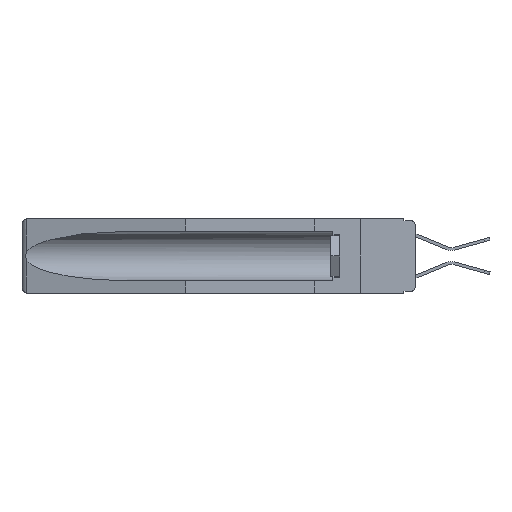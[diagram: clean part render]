
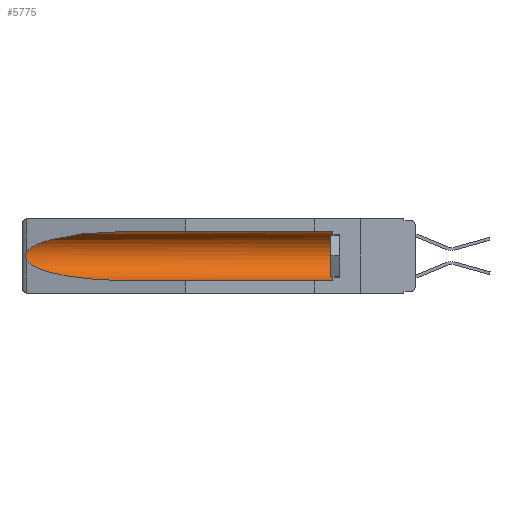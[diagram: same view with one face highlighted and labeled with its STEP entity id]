
A CAD part, left-side view. The second image highlights one B-rep face of the part: STEP entity #5775.
In plain terms, the highlighted cylindrical face has radius 2.857 mm (diameter 5.715 mm), a partial arc.
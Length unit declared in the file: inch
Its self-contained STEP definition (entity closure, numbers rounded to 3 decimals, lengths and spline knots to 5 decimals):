
#430 = VECTOR ( 'NONE', #15503, 39.37008 ) ;
#991 = DIRECTION ( 'NONE',  ( 0., 1., 0. ) ) ;
#1153 = CARTESIAN_POINT ( 'NONE',  ( 0.26537, 1.52718, -0.14972 ) ) ;
#1721 = CARTESIAN_POINT ( 'NONE',  ( 0.2675, 1.53308, -0.16763 ) ) ;
#1985 = DIRECTION ( 'NONE',  ( 0., 0., 1. ) ) ;
#2194 = ORIENTED_EDGE ( 'NONE', *, *, #4719, .T. ) ;
#2524 = VERTEX_POINT ( 'NONE', #5177 ) ;
#2529 = VERTEX_POINT ( 'NONE', #14973 ) ;
#2589 = VECTOR ( 'NONE', #991, 39.37008 ) ;
#3140 = CARTESIAN_POINT ( 'NONE',  ( 0.26597, 1.5296, -0.19026 ) ) ;
#3975 = FACE_OUTER_BOUND ( 'NONE', #15320, .T. ) ;
#4367 = CARTESIAN_POINT ( 'NONE',  ( 0.155, -0.30754, -0.284 ) ) ;
#4464 = CARTESIAN_POINT ( 'NONE',  ( 0.155, -0.30754, -0.059 ) ) ;
#4719 = EDGE_CURVE ( 'NONE', #2524, #11640, #8384, .T. ) ;
#4727 = LINE ( 'NONE', #4367, #430 ) ;
#5177 = CARTESIAN_POINT ( 'NONE',  ( 0.155, 1.07973, -0.059 ) ) ;
#5775 = ADVANCED_FACE ( 'NONE', ( #3975 ), #19039, .F. ) ;
#5971 = EDGE_CURVE ( 'NONE', #19521, #2529, #4727, .T. ) ;
#6117 = CARTESIAN_POINT ( 'NONE',  ( 0.155, -0.30754, -0.1715 ) ) ;
#6275 = CARTESIAN_POINT ( 'NONE',  ( 0.26655, 1.53094, -0.18657 ) ) ;
#6411 = CARTESIAN_POINT ( 'NONE',  ( 0.26597, 1.52961, -0.15275 ) ) ;
#6857 = CARTESIAN_POINT ( 'NONE',  ( 0.155, 0.126, -0.1715 ) ) ;
#6981 = EDGE_CURVE ( 'NONE', #19657, #2529, #10424, .T. ) ;
#8384 =( BOUNDED_CURVE ( )  B_SPLINE_CURVE ( 3, ( #14329, #19924, #10711, #1153 ),
 .UNSPECIFIED., .F., .F. ) 
 B_SPLINE_CURVE_WITH_KNOTS ( ( 4, 4 ),
 ( 4.71239, 6.08839 ),
 .UNSPECIFIED. ) 
 CURVE ( )  GEOMETRIC_REPRESENTATION_ITEM ( )  RATIONAL_B_SPLINE_CURVE ( ( 1., 0.848, 0.848, 1. ) ) 
 REPRESENTATION_ITEM ( '' )  );
#8856 = LINE ( 'NONE', #4464, #2589 ) ;
#9444 = CARTESIAN_POINT ( 'NONE',  ( 0.26537, 1.52718, -0.19328 ) ) ;
#9794 = B_SPLINE_CURVE_WITH_KNOTS ( 'NONE', 3,
 ( #15824, #6411, #12752, #19208, #1721, #19073, #12892, #6275, #3140, #9444 ),
 .UNSPECIFIED., .F., .F.,
 ( 4, 2, 2, 2, 4 ),
 ( 0., 0.00029, 0.00058, 0.00087, 0.00117 ),
 .UNSPECIFIED. ) ;
#9916 = ORIENTED_EDGE ( 'NONE', *, *, #14236, .T. ) ;
#10424 =( BOUNDED_CURVE ( )  B_SPLINE_CURVE ( 3, ( #15253, #15321, #13719, #15037 ),
 .UNSPECIFIED., .F., .F. ) 
 B_SPLINE_CURVE_WITH_KNOTS ( ( 4, 4 ),
 ( 0.1948, 1.5708 ),
 .UNSPECIFIED. ) 
 CURVE ( )  GEOMETRIC_REPRESENTATION_ITEM ( )  RATIONAL_B_SPLINE_CURVE ( ( 1., 0.848, 0.848, 1. ) ) 
 REPRESENTATION_ITEM ( '' )  );
#10683 = DIRECTION ( 'NONE',  ( 0., 1., 0. ) ) ;
#10711 = CARTESIAN_POINT ( 'NONE',  ( 0.25451, 1.48313, -0.09465 ) ) ;
#11528 = EDGE_CURVE ( 'NONE', #15801, #2524, #8856, .T. ) ;
#11640 = VERTEX_POINT ( 'NONE', #12591 ) ;
#12097 = CIRCLE ( 'NONE', #18278, 0.1125 ) ;
#12290 = DIRECTION ( 'NONE',  ( 0., 0., 1. ) ) ;
#12591 = CARTESIAN_POINT ( 'NONE',  ( 0.26537, 1.52718, -0.14972 ) ) ;
#12752 = CARTESIAN_POINT ( 'NONE',  ( 0.26654, 1.53092, -0.15636 ) ) ;
#12892 = CARTESIAN_POINT ( 'NONE',  ( 0.2673, 1.53269, -0.17917 ) ) ;
#13719 = CARTESIAN_POINT ( 'NONE',  ( 0.21114, 1.30732, -0.284 ) ) ;
#14004 = CARTESIAN_POINT ( 'NONE',  ( 0.155, 0.126, -0.059 ) ) ;
#14236 = EDGE_CURVE ( 'NONE', #11640, #19657, #9794, .T. ) ;
#14329 = CARTESIAN_POINT ( 'NONE',  ( 0.155, 1.07973, -0.059 ) ) ;
#14900 = CARTESIAN_POINT ( 'NONE',  ( 0.155, 0.126, -0.284 ) ) ;
#14973 = CARTESIAN_POINT ( 'NONE',  ( 0.155, 1.07973, -0.284 ) ) ;
#15037 = CARTESIAN_POINT ( 'NONE',  ( 0.155, 1.07973, -0.284 ) ) ;
#15091 = ORIENTED_EDGE ( 'NONE', *, *, #5971, .F. ) ;
#15253 = CARTESIAN_POINT ( 'NONE',  ( 0.26537, 1.52718, -0.19328 ) ) ;
#15320 = EDGE_LOOP ( 'NONE', ( #2194, #9916, #17595, #15091, #20447, #17634 ) ) ;
#15321 = CARTESIAN_POINT ( 'NONE',  ( 0.25451, 1.48313, -0.24835 ) ) ;
#15503 = DIRECTION ( 'NONE',  ( 0., 1., 0. ) ) ;
#15801 = VERTEX_POINT ( 'NONE', #14004 ) ;
#15824 = CARTESIAN_POINT ( 'NONE',  ( 0.26537, 1.52718, -0.14972 ) ) ;
#16727 = EDGE_CURVE ( 'NONE', #19521, #15801, #12097, .T. ) ;
#17595 = ORIENTED_EDGE ( 'NONE', *, *, #6981, .T. ) ;
#17634 = ORIENTED_EDGE ( 'NONE', *, *, #11528, .T. ) ;
#17843 = AXIS2_PLACEMENT_3D ( 'NONE', #6117, #10683, #12290 ) ;
#17988 = DIRECTION ( 'NONE',  ( 0., -1., 0. ) ) ;
#18278 = AXIS2_PLACEMENT_3D ( 'NONE', #6857, #17988, #1985 ) ;
#18517 = CARTESIAN_POINT ( 'NONE',  ( 0.26537, 1.52718, -0.19328 ) ) ;
#19039 = CYLINDRICAL_SURFACE ( 'NONE', #17843, 0.1125 ) ;
#19073 = CARTESIAN_POINT ( 'NONE',  ( 0.2675, 1.53308, -0.17534 ) ) ;
#19208 = CARTESIAN_POINT ( 'NONE',  ( 0.2673, 1.5327, -0.16383 ) ) ;
#19521 = VERTEX_POINT ( 'NONE', #14900 ) ;
#19657 = VERTEX_POINT ( 'NONE', #18517 ) ;
#19924 = CARTESIAN_POINT ( 'NONE',  ( 0.21114, 1.30732, -0.059 ) ) ;
#20447 = ORIENTED_EDGE ( 'NONE', *, *, #16727, .T. ) ;
